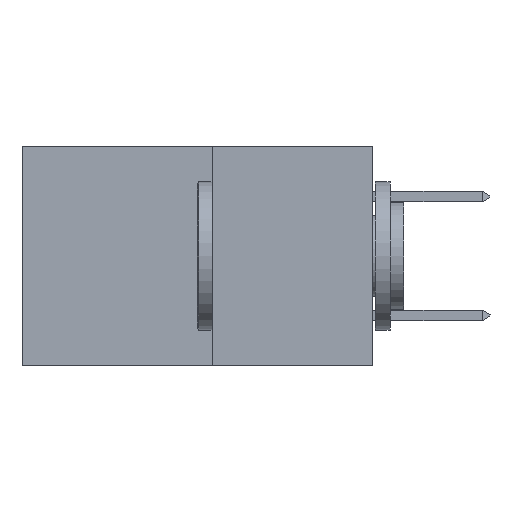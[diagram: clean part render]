
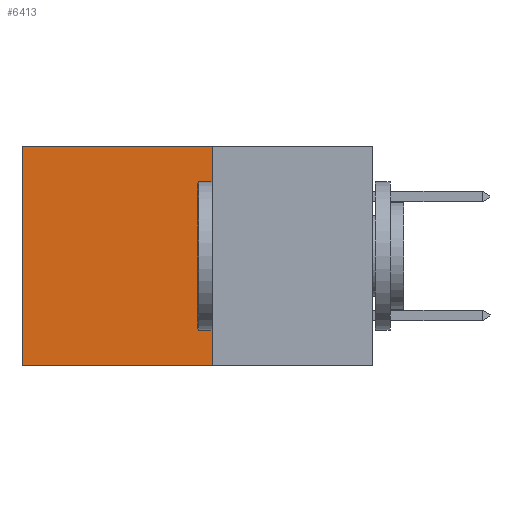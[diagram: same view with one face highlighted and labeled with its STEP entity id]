
A CAD part, left-side view. The second image highlights one B-rep face of the part: STEP entity #6413.
In plain terms, the highlighted planar face has unit normal (-1, 0, 0).
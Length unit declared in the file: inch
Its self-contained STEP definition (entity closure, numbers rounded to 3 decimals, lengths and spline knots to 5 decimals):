
#672 = LINE ( 'NONE', #22708, #25145 ) ;
#2414 = CARTESIAN_POINT ( 'NONE',  ( 0.277, 0.27, -0.37 ) ) ;
#3212 = VERTEX_POINT ( 'NONE', #13635 ) ;
#3429 = EDGE_CURVE ( 'NONE', #10055, #12898, #672, .T. ) ;
#3947 = EDGE_CURVE ( 'NONE', #9155, #12898, #17593, .T. ) ;
#4688 = ORIENTED_EDGE ( 'NONE', *, *, #26376, .T. ) ;
#6010 = VECTOR ( 'NONE', #9702, 39.37008 ) ;
#6413 = ADVANCED_FACE ( 'NONE', ( #28903 ), #13304, .F. ) ;
#6891 = LINE ( 'NONE', #18155, #29181 ) ;
#7218 = ORIENTED_EDGE ( 'NONE', *, *, #3947, .F. ) ;
#7597 = CARTESIAN_POINT ( 'NONE',  ( 0.277, 0.27, -0.37 ) ) ;
#8971 = ORIENTED_EDGE ( 'NONE', *, *, #11729, .F. ) ;
#9155 = VERTEX_POINT ( 'NONE', #2414 ) ;
#9702 = DIRECTION ( 'NONE',  ( 0., 1., 0. ) ) ;
#10055 = VERTEX_POINT ( 'NONE', #17307 ) ;
#11729 = EDGE_CURVE ( 'NONE', #3212, #9155, #6891, .T. ) ;
#12898 = VERTEX_POINT ( 'NONE', #16299 ) ;
#13129 = DIRECTION ( 'NONE',  ( 0., 0., -1. ) ) ;
#13136 = DIRECTION ( 'NONE',  ( 1., 0., 0. ) ) ;
#13201 = CARTESIAN_POINT ( 'NONE',  ( 0.277, 0.27, -0.37 ) ) ;
#13304 = PLANE ( 'NONE',  #20475 ) ;
#13635 = CARTESIAN_POINT ( 'NONE',  ( 0.277, 0.27, 0. ) ) ;
#14916 = LINE ( 'NONE', #25169, #26402 ) ;
#16299 = CARTESIAN_POINT ( 'NONE',  ( 0.277, 0.59, -0.37 ) ) ;
#17307 = CARTESIAN_POINT ( 'NONE',  ( 0.277, 0.59, 0. ) ) ;
#17593 = LINE ( 'NONE', #7597, #6010 ) ;
#18155 = CARTESIAN_POINT ( 'NONE',  ( 0.277, 0.27, -0.37 ) ) ;
#20456 = DIRECTION ( 'NONE',  ( 0., 0., -1. ) ) ;
#20475 = AXIS2_PLACEMENT_3D ( 'NONE', #13201, #13136, #13129 ) ;
#22412 = DIRECTION ( 'NONE',  ( 0., 0., -1. ) ) ;
#22708 = CARTESIAN_POINT ( 'NONE',  ( 0.277, 0.59, -0.37 ) ) ;
#25145 = VECTOR ( 'NONE', #22412, 39.37008 ) ;
#25169 = CARTESIAN_POINT ( 'NONE',  ( 0.277, 0.27, 0. ) ) ;
#25376 = ORIENTED_EDGE ( 'NONE', *, *, #3429, .T. ) ;
#26376 = EDGE_CURVE ( 'NONE', #3212, #10055, #14916, .T. ) ;
#26402 = VECTOR ( 'NONE', #27440, 39.37008 ) ;
#27166 = EDGE_LOOP ( 'NONE', ( #25376, #7218, #8971, #4688 ) ) ;
#27440 = DIRECTION ( 'NONE',  ( 0., 1., 0. ) ) ;
#28903 = FACE_OUTER_BOUND ( 'NONE', #27166, .T. ) ;
#29181 = VECTOR ( 'NONE', #20456, 39.37008 ) ;
